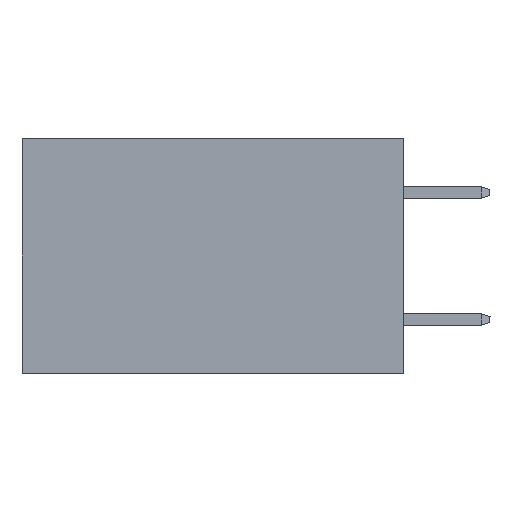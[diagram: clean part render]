
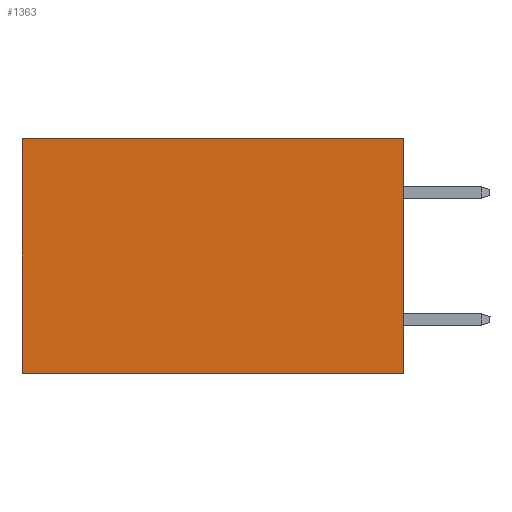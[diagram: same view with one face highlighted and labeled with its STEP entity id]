
A CAD part, left-side view. The second image highlights one B-rep face of the part: STEP entity #1363.
In plain terms, the highlighted planar face has unit normal (-1, 0, 0).
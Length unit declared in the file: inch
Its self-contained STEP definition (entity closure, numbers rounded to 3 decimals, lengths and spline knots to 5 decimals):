
#418 = VECTOR ( 'NONE', #3727, 39.37008 ) ;
#499 = EDGE_CURVE ( 'NONE', #1942, #2745, #4784, .T. ) ;
#1363 = ADVANCED_FACE ( 'NONE', ( #12364 ), #2722, .F. ) ;
#1942 = VERTEX_POINT ( 'NONE', #10671 ) ;
#2275 = ORIENTED_EDGE ( 'NONE', *, *, #10548, .F. ) ;
#2380 = VERTEX_POINT ( 'NONE', #3039 ) ;
#2722 = PLANE ( 'NONE',  #10527 ) ;
#2745 = VERTEX_POINT ( 'NONE', #3117 ) ;
#3039 = CARTESIAN_POINT ( 'NONE',  ( 0.2875, 0., -0.37 ) ) ;
#3117 = CARTESIAN_POINT ( 'NONE',  ( 0.2875, 0.6, 0. ) ) ;
#3198 = VECTOR ( 'NONE', #6029, 39.37008 ) ;
#3490 = ORIENTED_EDGE ( 'NONE', *, *, #499, .T. ) ;
#3727 = DIRECTION ( 'NONE',  ( 0., 1., 0. ) ) ;
#4006 = DIRECTION ( 'NONE',  ( 0., 0., -1. ) ) ;
#4784 = LINE ( 'NONE', #5895, #418 ) ;
#4832 = VECTOR ( 'NONE', #11181, 39.37008 ) ;
#4893 = LINE ( 'NONE', #11252, #4832 ) ;
#5895 = CARTESIAN_POINT ( 'NONE',  ( 0.2875, 0., 0. ) ) ;
#6029 = DIRECTION ( 'NONE',  ( 0., 0., -1. ) ) ;
#6100 = VECTOR ( 'NONE', #4006, 39.37008 ) ;
#6309 = LINE ( 'NONE', #7322, #3198 ) ;
#6529 = DIRECTION ( 'NONE',  ( 0., 0., -1. ) ) ;
#6812 = ORIENTED_EDGE ( 'NONE', *, *, #10484, .T. ) ;
#7322 = CARTESIAN_POINT ( 'NONE',  ( 0.2875, 0., 0. ) ) ;
#7728 = EDGE_CURVE ( 'NONE', #2380, #7943, #4893, .T. ) ;
#7943 = VERTEX_POINT ( 'NONE', #8495 ) ;
#8495 = CARTESIAN_POINT ( 'NONE',  ( 0.2875, 0.6, -0.37 ) ) ;
#9361 = CARTESIAN_POINT ( 'NONE',  ( 0.2875, 0.6, 0. ) ) ;
#10245 = CARTESIAN_POINT ( 'NONE',  ( 0.2875, 0., 0. ) ) ;
#10258 = EDGE_LOOP ( 'NONE', ( #6812, #12218, #2275, #3490 ) ) ;
#10484 = EDGE_CURVE ( 'NONE', #2745, #7943, #12670, .T. ) ;
#10527 = AXIS2_PLACEMENT_3D ( 'NONE', #10245, #13523, #6529 ) ;
#10548 = EDGE_CURVE ( 'NONE', #1942, #2380, #6309, .T. ) ;
#10671 = CARTESIAN_POINT ( 'NONE',  ( 0.2875, 0., 0. ) ) ;
#11181 = DIRECTION ( 'NONE',  ( 0., 1., 0. ) ) ;
#11252 = CARTESIAN_POINT ( 'NONE',  ( 0.2875, 0., -0.37 ) ) ;
#12218 = ORIENTED_EDGE ( 'NONE', *, *, #7728, .F. ) ;
#12364 = FACE_OUTER_BOUND ( 'NONE', #10258, .T. ) ;
#12670 = LINE ( 'NONE', #9361, #6100 ) ;
#13523 = DIRECTION ( 'NONE',  ( 1., 0., 0. ) ) ;
